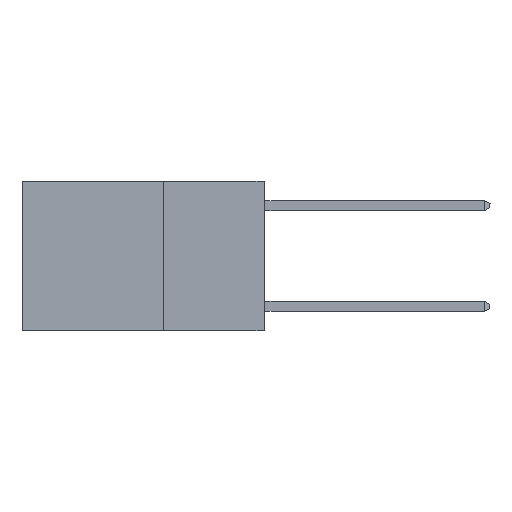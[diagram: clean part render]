
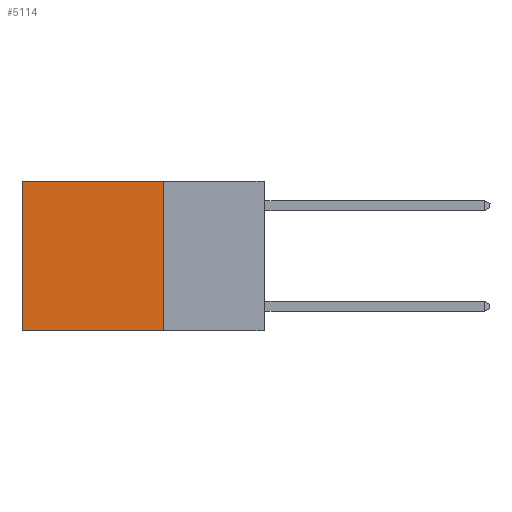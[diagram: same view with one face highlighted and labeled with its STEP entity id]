
A CAD part, left-side view. The second image highlights one B-rep face of the part: STEP entity #5114.
In plain terms, the highlighted planar face has unit normal (-1, 0, 0).
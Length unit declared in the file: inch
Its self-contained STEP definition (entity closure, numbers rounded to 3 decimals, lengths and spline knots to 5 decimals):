
#485 = VERTEX_POINT ( 'NONE', #14257 ) ;
#2651 = LINE ( 'NONE', #5804, #12146 ) ;
#4158 = ORIENTED_EDGE ( 'NONE', *, *, #8031, .T. ) ;
#5114 = ADVANCED_FACE ( 'NONE', ( #18626 ), #14472, .F. ) ;
#5349 = DIRECTION ( 'NONE',  ( 0., 0., -1. ) ) ;
#5804 = CARTESIAN_POINT ( 'NONE',  ( 0.2625, 0.25, -0.37 ) ) ;
#6229 = CARTESIAN_POINT ( 'NONE',  ( 0.2625, 0.25, 0. ) ) ;
#6531 = CARTESIAN_POINT ( 'NONE',  ( 0.2625, 0.6, 0. ) ) ;
#7422 = LINE ( 'NONE', #6229, #21938 ) ;
#8031 = EDGE_CURVE ( 'NONE', #10604, #16186, #19714, .T. ) ;
#8337 = EDGE_CURVE ( 'NONE', #19529, #485, #18802, .T. ) ;
#8448 = DIRECTION ( 'NONE',  ( 0., 0., -1. ) ) ;
#8675 = CARTESIAN_POINT ( 'NONE',  ( 0.2625, 0.25, 0. ) ) ;
#10604 = VERTEX_POINT ( 'NONE', #20817 ) ;
#11041 = CARTESIAN_POINT ( 'NONE',  ( 0.2625, 0.6, -0.37 ) ) ;
#12146 = VECTOR ( 'NONE', #17147, 39.37008 ) ;
#12646 = DIRECTION ( 'NONE',  ( 0., 0., -1. ) ) ;
#14257 = CARTESIAN_POINT ( 'NONE',  ( 0.2625, 0.25, -0.37 ) ) ;
#14472 = PLANE ( 'NONE',  #23462 ) ;
#14696 = ORIENTED_EDGE ( 'NONE', *, *, #18464, .T. ) ;
#15742 = DIRECTION ( 'NONE',  ( 0., 1., 0. ) ) ;
#16186 = VERTEX_POINT ( 'NONE', #11041 ) ;
#17147 = DIRECTION ( 'NONE',  ( 0., 1., 0. ) ) ;
#17978 = ORIENTED_EDGE ( 'NONE', *, *, #24428, .F. ) ;
#18464 = EDGE_CURVE ( 'NONE', #19529, #10604, #7422, .T. ) ;
#18626 = FACE_OUTER_BOUND ( 'NONE', #23460, .T. ) ;
#18802 = LINE ( 'NONE', #24176, #19406 ) ;
#19406 = VECTOR ( 'NONE', #5349, 39.37008 ) ;
#19529 = VERTEX_POINT ( 'NONE', #22782 ) ;
#19714 = LINE ( 'NONE', #6531, #24092 ) ;
#20817 = CARTESIAN_POINT ( 'NONE',  ( 0.2625, 0.6, 0. ) ) ;
#21938 = VECTOR ( 'NONE', #15742, 39.37008 ) ;
#22782 = CARTESIAN_POINT ( 'NONE',  ( 0.2625, 0.25, 0. ) ) ;
#23078 = ORIENTED_EDGE ( 'NONE', *, *, #8337, .F. ) ;
#23460 = EDGE_LOOP ( 'NONE', ( #4158, #17978, #23078, #14696 ) ) ;
#23462 = AXIS2_PLACEMENT_3D ( 'NONE', #8675, #23928, #12646 ) ;
#23928 = DIRECTION ( 'NONE',  ( 1., 0., 0. ) ) ;
#24092 = VECTOR ( 'NONE', #8448, 39.37008 ) ;
#24176 = CARTESIAN_POINT ( 'NONE',  ( 0.2625, 0.25, 0. ) ) ;
#24428 = EDGE_CURVE ( 'NONE', #485, #16186, #2651, .T. ) ;
